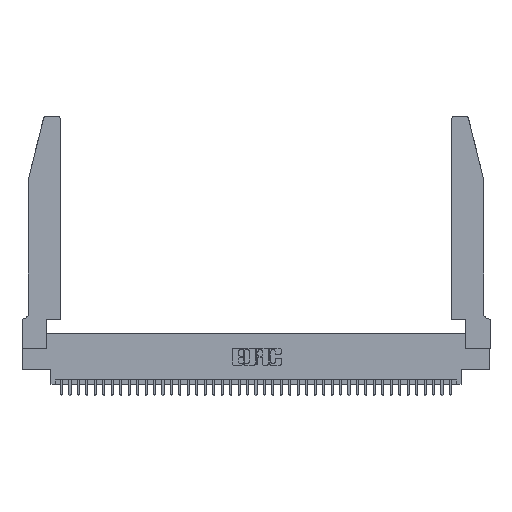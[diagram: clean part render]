
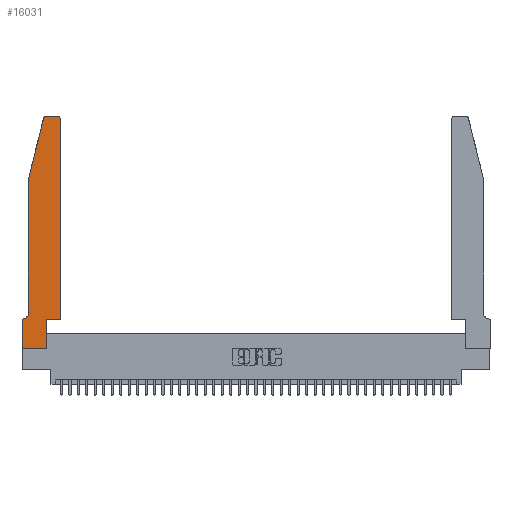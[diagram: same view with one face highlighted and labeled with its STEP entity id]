
A CAD part, top view. The second image highlights one B-rep face of the part: STEP entity #16031.
In plain terms, the highlighted planar face has unit normal (0, 0, 1).
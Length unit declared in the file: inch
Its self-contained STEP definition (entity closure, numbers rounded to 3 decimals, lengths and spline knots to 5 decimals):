
#64 = VERTEX_POINT ( 'NONE', #13925 ) ;
#371 = VERTEX_POINT ( 'NONE', #27838 ) ;
#436 = DIRECTION ( 'NONE',  ( 1., 0., 0. ) ) ;
#579 = CARTESIAN_POINT ( 'NONE',  ( 0.4505, 0.35, 0.37 ) ) ;
#1375 = CARTESIAN_POINT ( 'NONE',  ( 0., 0., 0.37 ) ) ;
#1566 = DIRECTION ( 'NONE',  ( 0., -1., 0. ) ) ;
#1582 = EDGE_CURVE ( 'NONE', #28195, #15845, #9542, .T. ) ;
#1638 = VECTOR ( 'NONE', #26181, 39.37008 ) ;
#2499 = DIRECTION ( 'NONE',  ( -1., 0., 0. ) ) ;
#2572 = CIRCLE ( 'NONE', #23812, 0.03 ) ;
#2810 = LINE ( 'NONE', #6563, #11417 ) ;
#3045 = CARTESIAN_POINT ( 'NONE',  ( 0.284, 2.75, 0.37 ) ) ;
#3339 = EDGE_CURVE ( 'NONE', #17910, #24978, #11282, .T. ) ;
#4885 = CARTESIAN_POINT ( 'NONE',  ( 0.2865, 0.35, 0.37 ) ) ;
#6119 = ORIENTED_EDGE ( 'NONE', *, *, #21403, .T. ) ;
#6131 = VERTEX_POINT ( 'NONE', #38806 ) ;
#6563 = CARTESIAN_POINT ( 'NONE',  ( 0.2605, 2.75, 0.37 ) ) ;
#7285 = CARTESIAN_POINT ( 'NONE',  ( 0.4505, 2.72, 0.37 ) ) ;
#8190 = CIRCLE ( 'NONE', #15849, 0.03 ) ;
#8287 = EDGE_CURVE ( 'NONE', #9825, #40771, #24023, .T. ) ;
#8673 = AXIS2_PLACEMENT_3D ( 'NONE', #38538, #19669, #436 ) ;
#9117 = LINE ( 'NONE', #31165, #40725 ) ;
#9542 = LINE ( 'NONE', #27199, #41124 ) ;
#9588 = VECTOR ( 'NONE', #25162, 39.37008 ) ;
#9825 = VERTEX_POINT ( 'NONE', #36607 ) ;
#10073 = EDGE_LOOP ( 'NONE', ( #15130, #21482, #39736, #27431, #17552, #12110, #13649, #25013, #17111, #6119, #11259, #31578 ) ) ;
#10582 = CARTESIAN_POINT ( 'NONE',  ( 0.284, 2.72, 0.37 ) ) ;
#11259 = ORIENTED_EDGE ( 'NONE', *, *, #3339, .T. ) ;
#11282 = LINE ( 'NONE', #579, #1638 ) ;
#11353 = CARTESIAN_POINT ( 'NONE',  ( 0., 0., 0.37 ) ) ;
#11417 = VECTOR ( 'NONE', #19371, 39.37008 ) ;
#12110 = ORIENTED_EDGE ( 'NONE', *, *, #30024, .T. ) ;
#12347 = EDGE_CURVE ( 'NONE', #40771, #6131, #37510, .T. ) ;
#13649 = ORIENTED_EDGE ( 'NONE', *, *, #8287, .T. ) ;
#13828 = DIRECTION ( 'NONE',  ( 1., 0., 0. ) ) ;
#13925 = CARTESIAN_POINT ( 'NONE',  ( 0.4205, 2.75, 0.37 ) ) ;
#14529 = DIRECTION ( 'NONE',  ( 0., 0., 1. ) ) ;
#15130 = ORIENTED_EDGE ( 'NONE', *, *, #33126, .T. ) ;
#15445 = DIRECTION ( 'NONE',  ( -1., 0., 0. ) ) ;
#15601 = VECTOR ( 'NONE', #1566, 39.37008 ) ;
#15845 = VERTEX_POINT ( 'NONE', #25101 ) ;
#15849 = AXIS2_PLACEMENT_3D ( 'NONE', #10582, #32700, #13828 ) ;
#16031 = ADVANCED_FACE ( 'NONE', ( #36839 ), #29081, .T. ) ;
#16067 = DIRECTION ( 'NONE',  ( 0., -1., 0. ) ) ;
#16069 = VECTOR ( 'NONE', #16067, 39.37008 ) ;
#17111 = ORIENTED_EDGE ( 'NONE', *, *, #31851, .T. ) ;
#17125 = CARTESIAN_POINT ( 'NONE',  ( 0.4505, 0.35, 0.37 ) ) ;
#17552 = ORIENTED_EDGE ( 'NONE', *, *, #20149, .T. ) ;
#17786 = DIRECTION ( 'NONE',  ( -0.239, -0.971, 0. ) ) ;
#17910 = VERTEX_POINT ( 'NONE', #17125 ) ;
#18044 = LINE ( 'NONE', #40933, #9588 ) ;
#18484 = CARTESIAN_POINT ( 'NONE',  ( 0.2865, 0.35, 0.37 ) ) ;
#19371 = DIRECTION ( 'NONE',  ( -1., 0., 0. ) ) ;
#19669 = DIRECTION ( 'NONE',  ( 0., 0., 1. ) ) ;
#20149 = EDGE_CURVE ( 'NONE', #371, #30244, #20710, .T. ) ;
#20710 = CIRCLE ( 'NONE', #29748, 0.07 ) ;
#20759 = VECTOR ( 'NONE', #23788, 39.37008 ) ;
#21403 = EDGE_CURVE ( 'NONE', #39826, #17910, #18044, .T. ) ;
#21482 = ORIENTED_EDGE ( 'NONE', *, *, #36805, .T. ) ;
#21683 = DIRECTION ( 'NONE',  ( 0., 0., -1. ) ) ;
#23492 = LINE ( 'NONE', #34948, #16069 ) ;
#23788 = DIRECTION ( 'NONE',  ( 1., 0., 0. ) ) ;
#23812 = AXIS2_PLACEMENT_3D ( 'NONE', #33399, #14529, #36571 ) ;
#23978 = CARTESIAN_POINT ( 'NONE',  ( 0., 0., 0.37 ) ) ;
#24005 = DIRECTION ( 'NONE',  ( 0., 1., 0. ) ) ;
#24023 = LINE ( 'NONE', #23978, #15601 ) ;
#24978 = VERTEX_POINT ( 'NONE', #7285 ) ;
#25013 = ORIENTED_EDGE ( 'NONE', *, *, #12347, .T. ) ;
#25101 = CARTESIAN_POINT ( 'NONE',  ( 0.0755, 2., 0.37 ) ) ;
#25162 = DIRECTION ( 'NONE',  ( 1., 0., 0. ) ) ;
#25845 = LINE ( 'NONE', #4885, #33225 ) ;
#26181 = DIRECTION ( 'NONE',  ( 0., 1., 0. ) ) ;
#27199 = CARTESIAN_POINT ( 'NONE',  ( 0.0755, 2., 0.37 ) ) ;
#27238 = EDGE_CURVE ( 'NONE', #24978, #64, #2572, .T. ) ;
#27431 = ORIENTED_EDGE ( 'NONE', *, *, #37992, .T. ) ;
#27838 = CARTESIAN_POINT ( 'NONE',  ( 0.0755, 0.42, 0.37 ) ) ;
#28195 = VERTEX_POINT ( 'NONE', #34839 ) ;
#29081 = PLANE ( 'NONE',  #8673 ) ;
#29748 = AXIS2_PLACEMENT_3D ( 'NONE', #40509, #21683, #2499 ) ;
#30024 = EDGE_CURVE ( 'NONE', #30244, #9825, #9117, .T. ) ;
#30244 = VERTEX_POINT ( 'NONE', #35245 ) ;
#31165 = CARTESIAN_POINT ( 'NONE',  ( 0.0755, 0.35, 0.37 ) ) ;
#31578 = ORIENTED_EDGE ( 'NONE', *, *, #27238, .T. ) ;
#31851 = EDGE_CURVE ( 'NONE', #6131, #39826, #25845, .T. ) ;
#32700 = DIRECTION ( 'NONE',  ( 0., 0., 1. ) ) ;
#33126 = EDGE_CURVE ( 'NONE', #64, #37250, #2810, .T. ) ;
#33225 = VECTOR ( 'NONE', #24005, 39.37008 ) ;
#33399 = CARTESIAN_POINT ( 'NONE',  ( 0.4205, 2.72, 0.37 ) ) ;
#34839 = CARTESIAN_POINT ( 'NONE',  ( 0.25487, 2.72718, 0.37 ) ) ;
#34948 = CARTESIAN_POINT ( 'NONE',  ( 0.0755, 2., 0.37 ) ) ;
#35245 = CARTESIAN_POINT ( 'NONE',  ( 0.0055, 0.35, 0.37 ) ) ;
#36571 = DIRECTION ( 'NONE',  ( 1., 0., 0. ) ) ;
#36607 = CARTESIAN_POINT ( 'NONE',  ( 0., 0.35, 0.37 ) ) ;
#36805 = EDGE_CURVE ( 'NONE', #37250, #28195, #8190, .T. ) ;
#36839 = FACE_OUTER_BOUND ( 'NONE', #10073, .T. ) ;
#37250 = VERTEX_POINT ( 'NONE', #3045 ) ;
#37510 = LINE ( 'NONE', #1375, #20759 ) ;
#37992 = EDGE_CURVE ( 'NONE', #15845, #371, #23492, .T. ) ;
#38538 = CARTESIAN_POINT ( 'NONE',  ( 0., 0.35, 0.37 ) ) ;
#38806 = CARTESIAN_POINT ( 'NONE',  ( 0.2865, 0., 0.37 ) ) ;
#39736 = ORIENTED_EDGE ( 'NONE', *, *, #1582, .T. ) ;
#39826 = VERTEX_POINT ( 'NONE', #18484 ) ;
#40509 = CARTESIAN_POINT ( 'NONE',  ( 0.0055, 0.42, 0.37 ) ) ;
#40725 = VECTOR ( 'NONE', #15445, 39.37008 ) ;
#40771 = VERTEX_POINT ( 'NONE', #11353 ) ;
#40933 = CARTESIAN_POINT ( 'NONE',  ( 0.4505, 0.35, 0.37 ) ) ;
#41124 = VECTOR ( 'NONE', #17786, 39.37008 ) ;
